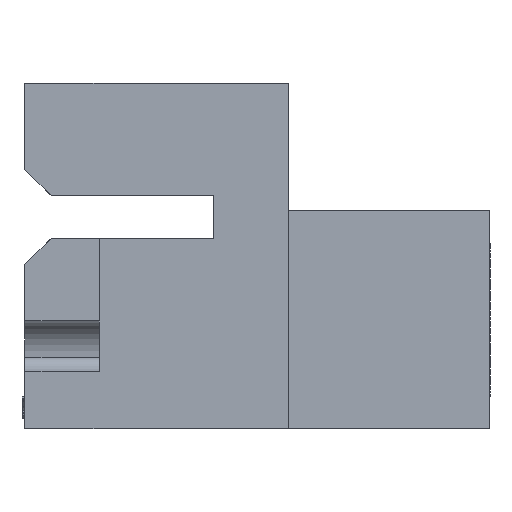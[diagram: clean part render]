
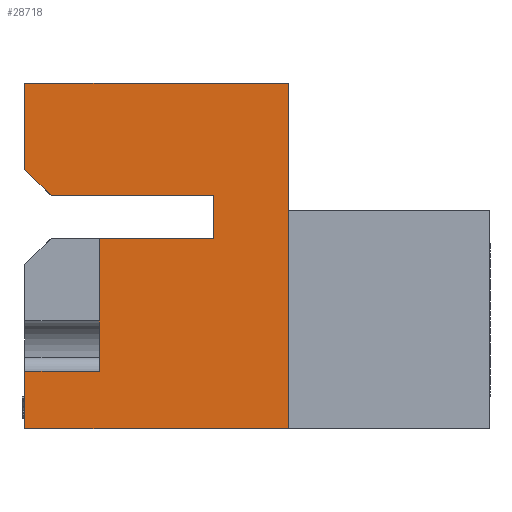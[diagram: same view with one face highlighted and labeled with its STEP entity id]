
A CAD part, left-side view. The second image highlights one B-rep face of the part: STEP entity #28718.
In plain terms, the highlighted planar face has unit normal (-1, 0, 0).
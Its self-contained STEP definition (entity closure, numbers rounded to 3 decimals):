
#1202 = LINE ( 'NONE', #42042, #27628 ) ;
#1212 = VERTEX_POINT ( 'NONE', #6353 ) ;
#1725 = CARTESIAN_POINT ( 'NONE',  ( 0., 11.506, -15.088 ) ) ;
#1937 = VECTOR ( 'NONE', #2954, 1000. ) ;
#2110 = VERTEX_POINT ( 'NONE', #40698 ) ;
#2264 = CARTESIAN_POINT ( 'NONE',  ( 0., 11.506, 0. ) ) ;
#2954 = DIRECTION ( 'NONE',  ( 0., 1., 0. ) ) ;
#3355 = ORIENTED_EDGE ( 'NONE', *, *, #12323, .F. ) ;
#3619 = CARTESIAN_POINT ( 'NONE',  ( 0., 0., -15.088 ) ) ;
#3787 = ORIENTED_EDGE ( 'NONE', *, *, #33226, .F. ) ;
#4098 = ORIENTED_EDGE ( 'NONE', *, *, #40471, .F. ) ;
#5569 = LINE ( 'NONE', #17464, #12390 ) ;
#5954 = LINE ( 'NONE', #33424, #24948 ) ;
#6353 = CARTESIAN_POINT ( 'NONE',  ( 0., 3.251, -6.782 ) ) ;
#6385 = DIRECTION ( 'NONE',  ( 0., -0.707, -0.707 ) ) ;
#7050 = EDGE_CURVE ( 'NONE', #1212, #20734, #40871, .T. ) ;
#7051 = ORIENTED_EDGE ( 'NONE', *, *, #23379, .F. ) ;
#7138 = DIRECTION ( 'NONE',  ( 0., 1., 0. ) ) ;
#7763 = CARTESIAN_POINT ( 'NONE',  ( 0., 0., -4.902 ) ) ;
#8439 = VECTOR ( 'NONE', #24498, 1000. ) ;
#9775 = VERTEX_POINT ( 'NONE', #23155 ) ;
#10166 = ORIENTED_EDGE ( 'NONE', *, *, #32413, .F. ) ;
#11149 = ORIENTED_EDGE ( 'NONE', *, *, #47062, .F. ) ;
#12323 = EDGE_CURVE ( 'NONE', #41375, #34055, #39733, .T. ) ;
#12390 = VECTOR ( 'NONE', #6385, 1000. ) ;
#12967 = ORIENTED_EDGE ( 'NONE', *, *, #17305, .T. ) ;
#14009 = DIRECTION ( 'NONE',  ( 0., 0., 1. ) ) ;
#14069 = LINE ( 'NONE', #1725, #35329 ) ;
#14339 = VECTOR ( 'NONE', #14009, 1000. ) ;
#15330 = CARTESIAN_POINT ( 'NONE',  ( 0., 8.255, -12.58 ) ) ;
#16035 = CARTESIAN_POINT ( 'NONE',  ( 0., 3.251, -4.902 ) ) ;
#16093 = CARTESIAN_POINT ( 'NONE',  ( 0., 8.255, -6.782 ) ) ;
#16113 = ORIENTED_EDGE ( 'NONE', *, *, #38380, .F. ) ;
#16153 = VERTEX_POINT ( 'NONE', #15330 ) ;
#17305 = EDGE_CURVE ( 'NONE', #16153, #29504, #27227, .T. ) ;
#17464 = CARTESIAN_POINT ( 'NONE',  ( 0., 10.363, -4.902 ) ) ;
#17906 = DIRECTION ( 'NONE',  ( 0., 0., 1. ) ) ;
#18446 = VECTOR ( 'NONE', #28554, 1000. ) ;
#20734 = VERTEX_POINT ( 'NONE', #16035 ) ;
#20803 = CARTESIAN_POINT ( 'NONE',  ( 0., -8.814, -15.088 ) ) ;
#20986 = CARTESIAN_POINT ( 'NONE',  ( 0., 11.506, -15.088 ) ) ;
#21398 = CARTESIAN_POINT ( 'NONE',  ( 0., 11.506, -12.58 ) ) ;
#21558 = CARTESIAN_POINT ( 'NONE',  ( 0., 8.255, -12.58 ) ) ;
#21829 = EDGE_CURVE ( 'NONE', #36556, #26366, #5569, .T. ) ;
#21903 = DIRECTION ( 'NONE',  ( 1., 0., 0. ) ) ;
#23155 = CARTESIAN_POINT ( 'NONE',  ( 0., 11.506, -15.088 ) ) ;
#23379 = EDGE_CURVE ( 'NONE', #9775, #29504, #14069, .T. ) ;
#23672 = VERTEX_POINT ( 'NONE', #3619 ) ;
#24316 = DIRECTION ( 'NONE',  ( 0., -1., 0. ) ) ;
#24498 = DIRECTION ( 'NONE',  ( 0., 1., 0. ) ) ;
#24557 = LINE ( 'NONE', #20803, #8439 ) ;
#24795 = EDGE_CURVE ( 'NONE', #34055, #23672, #5954, .T. ) ;
#24948 = VECTOR ( 'NONE', #30835, 1000. ) ;
#26366 = VERTEX_POINT ( 'NONE', #43504 ) ;
#27227 = LINE ( 'NONE', #21558, #1937 ) ;
#27398 = DIRECTION ( 'NONE',  ( 0., 0., 1. ) ) ;
#27628 = VECTOR ( 'NONE', #24316, 1000. ) ;
#27910 = AXIS2_PLACEMENT_3D ( 'NONE', #40257, #21903, #37198 ) ;
#28554 = DIRECTION ( 'NONE',  ( 0., -1., 0. ) ) ;
#28718 = ADVANCED_FACE ( 'NONE', ( #30487 ), #40599, .F. ) ;
#29504 = VERTEX_POINT ( 'NONE', #21398 ) ;
#29512 = ORIENTED_EDGE ( 'NONE', *, *, #24795, .F. ) ;
#30419 = DIRECTION ( 'NONE',  ( 0., 0., 1. ) ) ;
#30487 = FACE_OUTER_BOUND ( 'NONE', #44920, .T. ) ;
#30835 = DIRECTION ( 'NONE',  ( 0., 0., -1. ) ) ;
#31716 = VECTOR ( 'NONE', #30419, 1000. ) ;
#32277 = LINE ( 'NONE', #16093, #31716 ) ;
#32413 = EDGE_CURVE ( 'NONE', #20734, #26366, #43344, .T. ) ;
#32935 = VECTOR ( 'NONE', #7138, 1000. ) ;
#33226 = EDGE_CURVE ( 'NONE', #16153, #2110, #32277, .T. ) ;
#33424 = CARTESIAN_POINT ( 'NONE',  ( 0., 0., 0. ) ) ;
#34055 = VERTEX_POINT ( 'NONE', #47519 ) ;
#34967 = CARTESIAN_POINT ( 'NONE',  ( 0., 11.506, 0. ) ) ;
#35329 = VECTOR ( 'NONE', #27398, 1000. ) ;
#35375 = ORIENTED_EDGE ( 'NONE', *, *, #7050, .F. ) ;
#36556 = VERTEX_POINT ( 'NONE', #37715 ) ;
#36563 = ORIENTED_EDGE ( 'NONE', *, *, #21829, .T. ) ;
#37198 = DIRECTION ( 'NONE',  ( 0., 0., -1. ) ) ;
#37227 = VECTOR ( 'NONE', #17906, 1000. ) ;
#37715 = CARTESIAN_POINT ( 'NONE',  ( 0., 11.506, -3.759 ) ) ;
#38380 = EDGE_CURVE ( 'NONE', #23672, #9775, #24557, .T. ) ;
#39733 = LINE ( 'NONE', #2264, #18446 ) ;
#39938 = CARTESIAN_POINT ( 'NONE',  ( 0., 3.251, -6.782 ) ) ;
#40257 = CARTESIAN_POINT ( 'NONE',  ( 0., 0., 0. ) ) ;
#40471 = EDGE_CURVE ( 'NONE', #36556, #41375, #46968, .T. ) ;
#40599 = PLANE ( 'NONE',  #27910 ) ;
#40698 = CARTESIAN_POINT ( 'NONE',  ( 0., 8.255, -6.782 ) ) ;
#40871 = LINE ( 'NONE', #39938, #14339 ) ;
#41375 = VERTEX_POINT ( 'NONE', #34967 ) ;
#42042 = CARTESIAN_POINT ( 'NONE',  ( 0., 0., -6.782 ) ) ;
#43344 = LINE ( 'NONE', #7763, #32935 ) ;
#43504 = CARTESIAN_POINT ( 'NONE',  ( 0., 10.363, -4.902 ) ) ;
#44920 = EDGE_LOOP ( 'NONE', ( #16113, #29512, #3355, #4098, #36563, #10166, #35375, #11149, #3787, #12967, #7051 ) ) ;
#46968 = LINE ( 'NONE', #20986, #37227 ) ;
#47062 = EDGE_CURVE ( 'NONE', #2110, #1212, #1202, .T. ) ;
#47519 = CARTESIAN_POINT ( 'NONE',  ( 0., 0., 0. ) ) ;
